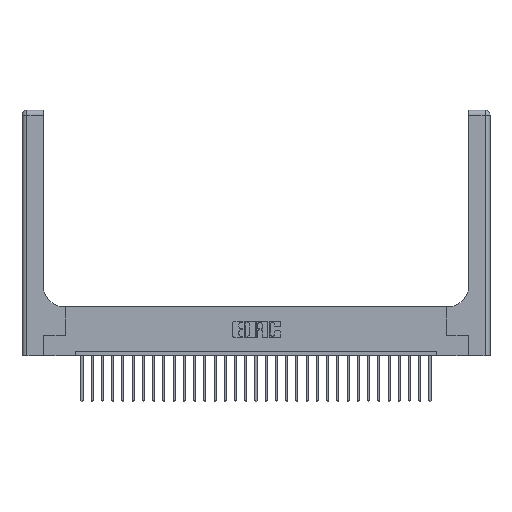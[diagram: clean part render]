
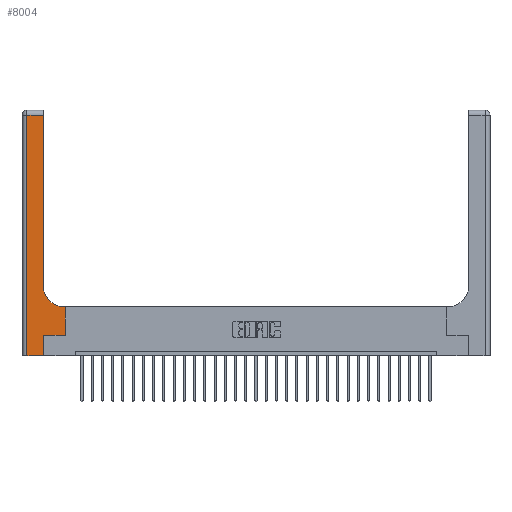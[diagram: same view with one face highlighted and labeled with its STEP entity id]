
A CAD part, top view. The second image highlights one B-rep face of the part: STEP entity #8004.
In plain terms, the highlighted planar face has unit normal (0, 0, 1).
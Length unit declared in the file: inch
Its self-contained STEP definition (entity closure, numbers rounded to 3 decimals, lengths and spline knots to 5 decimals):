
#33 = ORIENTED_EDGE ( 'NONE', *, *, #25717, .T. ) ;
#132 = ORIENTED_EDGE ( 'NONE', *, *, #3143, .T. ) ;
#185 = EDGE_CURVE ( 'NONE', #2663, #7492, #22304, .T. ) ;
#190 = VECTOR ( 'NONE', #11060, 39.37008 ) ;
#204 = CARTESIAN_POINT ( 'NONE',  ( 0.06, 2.94, 0.37 ) ) ;
#248 = ORIENTED_EDGE ( 'NONE', *, *, #18954, .T. ) ;
#345 = CARTESIAN_POINT ( 'NONE',  ( 0.265, 0., 0.37 ) ) ;
#659 = ORIENTED_EDGE ( 'NONE', *, *, #26945, .T. ) ;
#1155 = DIRECTION ( 'NONE',  ( 1., 0., 0. ) ) ;
#2284 = DIRECTION ( 'NONE',  ( 0., 1., 0. ) ) ;
#2363 = DIRECTION ( 'NONE',  ( -1., 0., 0. ) ) ;
#2468 = CARTESIAN_POINT ( 'NONE',  ( 0.51, 0.6, 0.37 ) ) ;
#2531 = LINE ( 'NONE', #25796, #22023 ) ;
#2657 = CARTESIAN_POINT ( 'NONE',  ( 0., 2.94, 0.37 ) ) ;
#2663 = VERTEX_POINT ( 'NONE', #7852 ) ;
#2903 = VERTEX_POINT ( 'NONE', #204 ) ;
#2930 = ORIENTED_EDGE ( 'NONE', *, *, #20607, .T. ) ;
#2954 = VECTOR ( 'NONE', #25883, 39.37008 ) ;
#3143 = EDGE_CURVE ( 'NONE', #7492, #20524, #22465, .T. ) ;
#3293 = VERTEX_POINT ( 'NONE', #26593 ) ;
#3435 = ORIENTED_EDGE ( 'NONE', *, *, #26503, .T. ) ;
#3570 = LINE ( 'NONE', #2657, #190 ) ;
#3770 = DIRECTION ( 'NONE',  ( -1., 0., 0. ) ) ;
#4407 = CARTESIAN_POINT ( 'NONE',  ( 0., 3., 0.37 ) ) ;
#4420 = VERTEX_POINT ( 'NONE', #9565 ) ;
#4437 = DIRECTION ( 'NONE',  ( 0., -1., 0. ) ) ;
#4545 = VECTOR ( 'NONE', #9910, 39.37008 ) ;
#5967 = EDGE_CURVE ( 'NONE', #20627, #3293, #8551, .T. ) ;
#6094 = VECTOR ( 'NONE', #3770, 39.37008 ) ;
#6940 = VERTEX_POINT ( 'NONE', #345 ) ;
#7359 = CARTESIAN_POINT ( 'NONE',  ( 0.528, 0.25, 0.37 ) ) ;
#7492 = VERTEX_POINT ( 'NONE', #7359 ) ;
#7852 = CARTESIAN_POINT ( 'NONE',  ( 0.265, 0.25, 0.37 ) ) ;
#8004 = ADVANCED_FACE ( 'NONE', ( #10549 ), #25864, .F. ) ;
#8028 = AXIS2_PLACEMENT_3D ( 'NONE', #4407, #27710, #2363 ) ;
#8165 = LINE ( 'NONE', #17565, #18341 ) ;
#8250 = ORIENTED_EDGE ( 'NONE', *, *, #185, .T. ) ;
#8285 = VECTOR ( 'NONE', #12959, 39.37008 ) ;
#8551 = CIRCLE ( 'NONE', #15206, 0.25 ) ;
#8586 = DIRECTION ( 'NONE',  ( 1., 0., 0. ) ) ;
#8655 = VERTEX_POINT ( 'NONE', #11936 ) ;
#9565 = CARTESIAN_POINT ( 'NONE',  ( 0.26, 2.94, 0.37 ) ) ;
#9910 = DIRECTION ( 'NONE',  ( 0., 1., 0. ) ) ;
#10549 = FACE_OUTER_BOUND ( 'NONE', #19727, .T. ) ;
#11060 = DIRECTION ( 'NONE',  ( -1., 0., 0. ) ) ;
#11936 = CARTESIAN_POINT ( 'NONE',  ( 0.06, 0., 0.37 ) ) ;
#12959 = DIRECTION ( 'NONE',  ( 1., 0., 0. ) ) ;
#14441 = ORIENTED_EDGE ( 'NONE', *, *, #5967, .T. ) ;
#15206 = AXIS2_PLACEMENT_3D ( 'NONE', #22514, #16105, #1155 ) ;
#15986 = LINE ( 'NONE', #22790, #4545 ) ;
#16105 = DIRECTION ( 'NONE',  ( 0., 0., -1. ) ) ;
#16366 = CARTESIAN_POINT ( 'NONE',  ( 0.528, 0.25, 0.37 ) ) ;
#16991 = CARTESIAN_POINT ( 'NONE',  ( 0.26, 0.6, 0.37 ) ) ;
#17565 = CARTESIAN_POINT ( 'NONE',  ( 0.265, 0., 0.37 ) ) ;
#18341 = VECTOR ( 'NONE', #2284, 39.37008 ) ;
#18954 = EDGE_CURVE ( 'NONE', #6940, #2663, #8165, .T. ) ;
#19727 = EDGE_LOOP ( 'NONE', ( #659, #3435, #21314, #33, #248, #8250, #132, #2930, #14441 ) ) ;
#20524 = VERTEX_POINT ( 'NONE', #23155 ) ;
#20607 = EDGE_CURVE ( 'NONE', #20524, #20627, #26349, .T. ) ;
#20627 = VERTEX_POINT ( 'NONE', #2468 ) ;
#20960 = VECTOR ( 'NONE', #8586, 39.37008 ) ;
#21314 = ORIENTED_EDGE ( 'NONE', *, *, #25157, .T. ) ;
#21486 = CARTESIAN_POINT ( 'NONE',  ( 0.265, 0.25, 0.37 ) ) ;
#22023 = VECTOR ( 'NONE', #4437, 39.37008 ) ;
#22304 = LINE ( 'NONE', #21486, #20960 ) ;
#22465 = LINE ( 'NONE', #16366, #2954 ) ;
#22514 = CARTESIAN_POINT ( 'NONE',  ( 0.51, 0.85, 0.37 ) ) ;
#22790 = CARTESIAN_POINT ( 'NONE',  ( 0.26, 3., 0.37 ) ) ;
#23155 = CARTESIAN_POINT ( 'NONE',  ( 0.528, 0.6, 0.37 ) ) ;
#23684 = CARTESIAN_POINT ( 'NONE',  ( 0., 0., 0.37 ) ) ;
#25157 = EDGE_CURVE ( 'NONE', #2903, #8655, #2531, .T. ) ;
#25717 = EDGE_CURVE ( 'NONE', #8655, #6940, #26135, .T. ) ;
#25796 = CARTESIAN_POINT ( 'NONE',  ( 0.06, 3., 0.37 ) ) ;
#25864 = PLANE ( 'NONE',  #8028 ) ;
#25883 = DIRECTION ( 'NONE',  ( 0., 1., 0. ) ) ;
#26135 = LINE ( 'NONE', #23684, #8285 ) ;
#26349 = LINE ( 'NONE', #16991, #6094 ) ;
#26503 = EDGE_CURVE ( 'NONE', #4420, #2903, #3570, .T. ) ;
#26593 = CARTESIAN_POINT ( 'NONE',  ( 0.26, 0.85, 0.37 ) ) ;
#26945 = EDGE_CURVE ( 'NONE', #3293, #4420, #15986, .T. ) ;
#27710 = DIRECTION ( 'NONE',  ( 0., 0., -1. ) ) ;
